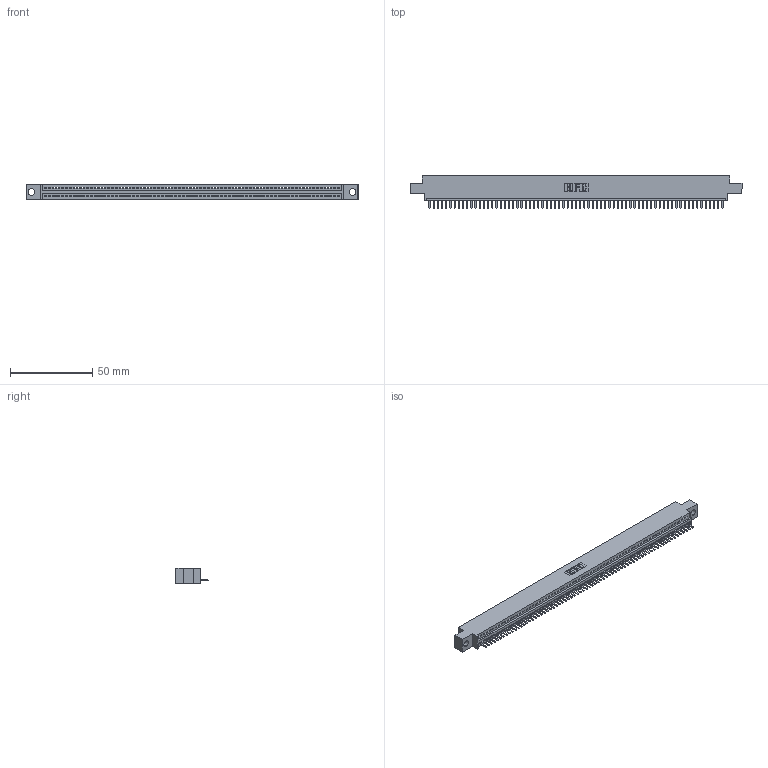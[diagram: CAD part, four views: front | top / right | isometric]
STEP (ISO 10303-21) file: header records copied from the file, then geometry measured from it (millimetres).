
FILE_DESCRIPTION (( 'STEP AP203' ), '1' );
FILE_NAME ('345-071-520-604.STEP', '2019-10-12T20:40:09', ( '' ), ( '' ), 'SwSTEP 2.0', 'SolidWorks 2016', '' );
FILE_SCHEMA (( 'CONFIG_CONTROL_DESIGN' ));
Length unit declared in the file: inch
Products named in the file (3): 345-292-001_345-293-120; 345 Part_0.170 Offset - 0.156 Dia-TH; 345-071-520-604
Assembly tree (72 placements, depth 2):
  345-071-520-604
    345 Part_0.170 Offset - 0.156 Dia-TH
    345-292-001_345-293-120  x71
Bounding box: 201.55 x 19.68 x 9.4 mm (x, y, z)
Volume: 18975.4 mm3; surface area: 24877.9 mm2
Topology: 72 solids, 72 shells, 4532 faces, 13417 edges, 8754 vertices
Faces by surface type: plane 3066, cylinder 1466
Entity records: 49781 total; most frequent: CARTESIAN_POINT 8641, ORIENTED_EDGE 8634, DIRECTION 7491, EDGE_CURVE 4317, VECTOR 3897, LINE 3897, VERTEX_POINT 2874, AXIS2_PLACEMENT_3D 1797
